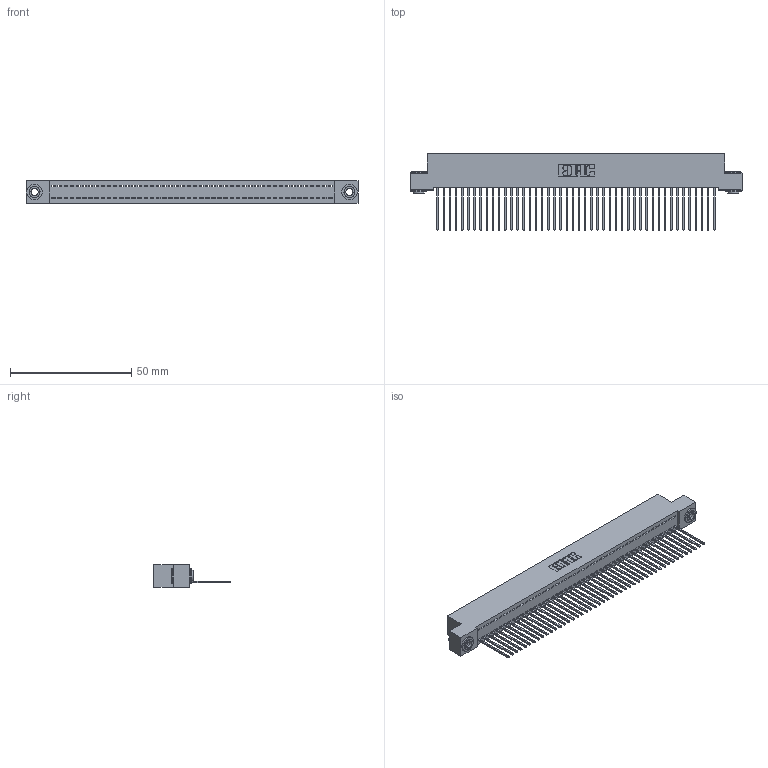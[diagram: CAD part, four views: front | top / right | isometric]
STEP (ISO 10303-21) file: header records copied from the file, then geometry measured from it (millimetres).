
FILE_DESCRIPTION (( 'STEP AP203' ), '1' );
FILE_NAME ('342-046-542-103.STEP', '2018-08-12T16:19:28', ( '' ), ( '' ), 'SwSTEP 2.0', 'SolidWorks 2016', '' );
FILE_SCHEMA (( 'CONFIG_CONTROL_DESIGN' ));
Length unit declared in the file: inch
Products named in the file (4): 345-292-001_345-293-142; 342-250-002_345-250-002-102; 342-046-542-103; 342 Part_.156 TH
Assembly tree (49 placements, depth 2):
  342-046-542-103
    342 Part_.156 TH
    345-292-001_345-293-142  x46
    342-250-002_345-250-002-102  x2
Bounding box: 137.16 x 31.63 x 9.4 mm (x, y, z)
Volume: 12166.1 mm3; surface area: 18790.4 mm2
Topology: 49 solids, 49 shells, 2816 faces, 8471 edges, 5582 vertices
Faces by surface type: plane 2008, cylinder 800, cone 8
Entity records: 28140 total; most frequent: CARTESIAN_POINT 4831, ORIENTED_EDGE 4806, DIRECTION 4101, EDGE_CURVE 2403, VECTOR 2251, LINE 2251, VERTEX_POINT 1598, AXIS2_PLACEMENT_3D 925
